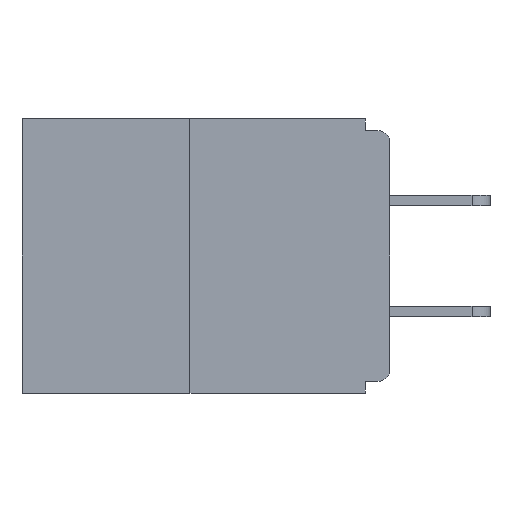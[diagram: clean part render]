
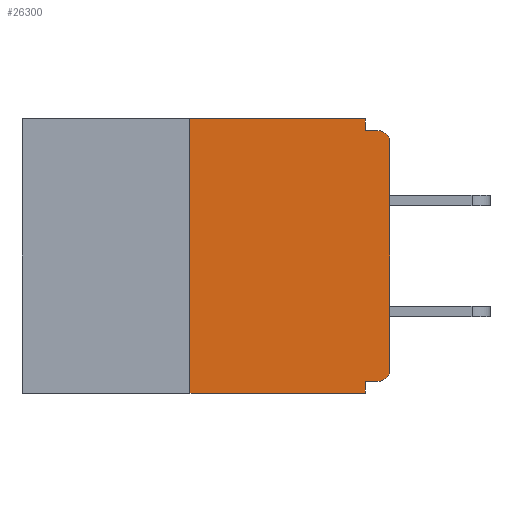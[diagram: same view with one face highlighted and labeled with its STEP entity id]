
A CAD part, left-side view. The second image highlights one B-rep face of the part: STEP entity #26300.
In plain terms, the highlighted planar face has unit normal (-1, 0, 0).
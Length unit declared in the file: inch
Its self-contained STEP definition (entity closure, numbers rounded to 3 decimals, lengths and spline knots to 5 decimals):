
#109 = ORIENTED_EDGE ( 'NONE', *, *, #15972, .T. ) ;
#167 = DIRECTION ( 'NONE',  ( 0., 0., -1. ) ) ;
#425 = FACE_OUTER_BOUND ( 'NONE', #13260, .T. ) ;
#454 = ORIENTED_EDGE ( 'NONE', *, *, #20028, .T. ) ;
#459 = LINE ( 'NONE', #2139, #15932 ) ;
#2139 = CARTESIAN_POINT ( 'NONE',  ( 0., 0., -0.015 ) ) ;
#2212 = EDGE_CURVE ( 'NONE', #22570, #6228, #18975, .T. ) ;
#2311 = LINE ( 'NONE', #12955, #24153 ) ;
#2913 = EDGE_CURVE ( 'NONE', #9569, #19608, #5043, .T. ) ;
#2914 = CARTESIAN_POINT ( 'NONE',  ( 0., 0., -0.328 ) ) ;
#2930 = ORIENTED_EDGE ( 'NONE', *, *, #11145, .F. ) ;
#3503 = VERTEX_POINT ( 'NONE', #5196 ) ;
#5043 = LINE ( 'NONE', #2914, #5721 ) ;
#5140 = DIRECTION ( 'NONE',  ( 0., 0., 1. ) ) ;
#5196 = CARTESIAN_POINT ( 'NONE',  ( 0., 0.25, 0. ) ) ;
#5625 = VECTOR ( 'NONE', #17216, 39.37008 ) ;
#5721 = VECTOR ( 'NONE', #7271, 39.37008 ) ;
#6228 = VERTEX_POINT ( 'NONE', #15251 ) ;
#6930 = LINE ( 'NONE', #19082, #5625 ) ;
#7004 = DIRECTION ( 'NONE',  ( 0., -1., 0. ) ) ;
#7271 = DIRECTION ( 'NONE',  ( 0., 1., 0. ) ) ;
#7278 = LINE ( 'NONE', #13540, #15161 ) ;
#7762 = DIRECTION ( 'NONE',  ( 0., -1., 0. ) ) ;
#7923 = CARTESIAN_POINT ( 'NONE',  ( 0., 0.25, 0. ) ) ;
#8643 = CARTESIAN_POINT ( 'NONE',  ( 0., 0., -0.03 ) ) ;
#9150 = DIRECTION ( 'NONE',  ( 0., 0., -1. ) ) ;
#9231 = CARTESIAN_POINT ( 'NONE',  ( 0., 0.25, -0.343 ) ) ;
#9499 = ORIENTED_EDGE ( 'NONE', *, *, #22583, .F. ) ;
#9569 = VERTEX_POINT ( 'NONE', #27113 ) ;
#10632 = CARTESIAN_POINT ( 'NONE',  ( 0., 0.015, -0.03 ) ) ;
#10962 = ORIENTED_EDGE ( 'NONE', *, *, #24706, .F. ) ;
#11145 = EDGE_CURVE ( 'NONE', #26407, #15042, #459, .T. ) ;
#12800 = LINE ( 'NONE', #7923, #25782 ) ;
#12955 = CARTESIAN_POINT ( 'NONE',  ( 0., 0., 0. ) ) ;
#13260 = EDGE_LOOP ( 'NONE', ( #9499, #10962, #23765, #23999, #24103, #454, #22095, #109, #2930, #17084 ) ) ;
#13288 = VERTEX_POINT ( 'NONE', #8643 ) ;
#13540 = CARTESIAN_POINT ( 'NONE',  ( 0., 0.031, 0. ) ) ;
#14081 = CARTESIAN_POINT ( 'NONE',  ( 0., 0.46, -0.343 ) ) ;
#14426 = CARTESIAN_POINT ( 'NONE',  ( 0., 0.015, -0.313 ) ) ;
#14816 = VERTEX_POINT ( 'NONE', #21332 ) ;
#14910 = CARTESIAN_POINT ( 'NONE',  ( 0., 0.031, -0.328 ) ) ;
#15042 = VERTEX_POINT ( 'NONE', #17846 ) ;
#15077 = AXIS2_PLACEMENT_3D ( 'NONE', #23916, #15239, #17544 ) ;
#15161 = VECTOR ( 'NONE', #9150, 39.37008 ) ;
#15239 = DIRECTION ( 'NONE',  ( 1., 0., 0. ) ) ;
#15251 = CARTESIAN_POINT ( 'NONE',  ( 0., 0.031, -0.343 ) ) ;
#15932 = VECTOR ( 'NONE', #16697, 39.37008 ) ;
#15972 = EDGE_CURVE ( 'NONE', #13288, #15042, #25589, .T. ) ;
#16107 = DIRECTION ( 'NONE',  ( 0., 0., -1. ) ) ;
#16697 = DIRECTION ( 'NONE',  ( 0., -1., 0. ) ) ;
#17084 = ORIENTED_EDGE ( 'NONE', *, *, #18059, .F. ) ;
#17216 = DIRECTION ( 'NONE',  ( 0., 0., -1. ) ) ;
#17544 = DIRECTION ( 'NONE',  ( 0., 0., -1. ) ) ;
#17846 = CARTESIAN_POINT ( 'NONE',  ( 0., 0.015, -0.015 ) ) ;
#18059 = EDGE_CURVE ( 'NONE', #24407, #26407, #7278, .T. ) ;
#18120 = DIRECTION ( 'NONE',  ( 0., 0., 1. ) ) ;
#18236 = CARTESIAN_POINT ( 'NONE',  ( 0., 0.031, -0.015 ) ) ;
#18299 = EDGE_CURVE ( 'NONE', #14816, #13288, #2311, .T. ) ;
#18975 = LINE ( 'NONE', #14081, #19959 ) ;
#19082 = CARTESIAN_POINT ( 'NONE',  ( 0., 0.031, -0.343 ) ) ;
#19403 = DIRECTION ( 'NONE',  ( -1., 0., 0. ) ) ;
#19499 = PLANE ( 'NONE',  #15077 ) ;
#19534 = LINE ( 'NONE', #26245, #24566 ) ;
#19608 = VERTEX_POINT ( 'NONE', #14910 ) ;
#19870 = AXIS2_PLACEMENT_3D ( 'NONE', #14426, #27301, #16107 ) ;
#19959 = VECTOR ( 'NONE', #7762, 39.37008 ) ;
#20028 = EDGE_CURVE ( 'NONE', #9569, #14816, #21404, .T. ) ;
#21332 = CARTESIAN_POINT ( 'NONE',  ( 0., 0., -0.313 ) ) ;
#21404 = CIRCLE ( 'NONE', #19870, 0.015 ) ;
#22095 = ORIENTED_EDGE ( 'NONE', *, *, #18299, .T. ) ;
#22570 = VERTEX_POINT ( 'NONE', #9231 ) ;
#22583 = EDGE_CURVE ( 'NONE', #3503, #24407, #19534, .T. ) ;
#23591 = AXIS2_PLACEMENT_3D ( 'NONE', #10632, #19403, #167 ) ;
#23765 = ORIENTED_EDGE ( 'NONE', *, *, #2212, .T. ) ;
#23916 = CARTESIAN_POINT ( 'NONE',  ( 0., 0.46, 0. ) ) ;
#23999 = ORIENTED_EDGE ( 'NONE', *, *, #24451, .F. ) ;
#24103 = ORIENTED_EDGE ( 'NONE', *, *, #2913, .F. ) ;
#24153 = VECTOR ( 'NONE', #5140, 39.37008 ) ;
#24407 = VERTEX_POINT ( 'NONE', #25060 ) ;
#24451 = EDGE_CURVE ( 'NONE', #19608, #6228, #6930, .T. ) ;
#24566 = VECTOR ( 'NONE', #7004, 39.37008 ) ;
#24706 = EDGE_CURVE ( 'NONE', #22570, #3503, #12800, .T. ) ;
#25060 = CARTESIAN_POINT ( 'NONE',  ( 0., 0.031, 0. ) ) ;
#25589 = CIRCLE ( 'NONE', #23591, 0.015 ) ;
#25782 = VECTOR ( 'NONE', #18120, 39.37008 ) ;
#26245 = CARTESIAN_POINT ( 'NONE',  ( 0., 0.46, 0. ) ) ;
#26300 = ADVANCED_FACE ( 'NONE', ( #425 ), #19499, .F. ) ;
#26407 = VERTEX_POINT ( 'NONE', #18236 ) ;
#27113 = CARTESIAN_POINT ( 'NONE',  ( 0., 0.015, -0.328 ) ) ;
#27301 = DIRECTION ( 'NONE',  ( -1., 0., 0. ) ) ;
